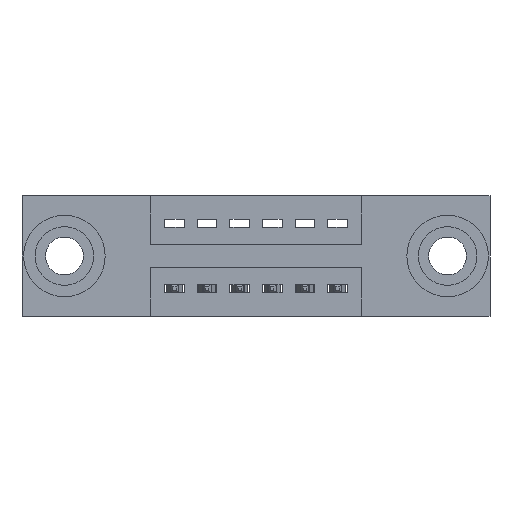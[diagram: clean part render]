
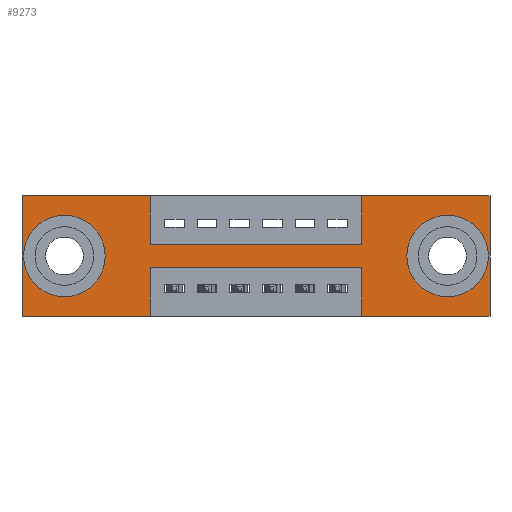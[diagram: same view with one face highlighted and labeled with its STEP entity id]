
A CAD part, front view. The second image highlights one B-rep face of the part: STEP entity #9273.
In plain terms, the highlighted planar face has unit normal (0, -1, 0).
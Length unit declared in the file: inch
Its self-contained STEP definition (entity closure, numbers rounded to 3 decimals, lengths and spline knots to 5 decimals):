
#13 = EDGE_CURVE ( 'NONE', #6455, #7511, #6539, .T. ) ;
#36 = ORIENTED_EDGE ( 'NONE', *, *, #2838, .F. ) ;
#334 = ORIENTED_EDGE ( 'NONE', *, *, #9604, .F. ) ;
#402 = DIRECTION ( 'NONE',  ( -1., 0., 0. ) ) ;
#462 = CARTESIAN_POINT ( 'NONE',  ( 0.3925, 0., -0.22 ) ) ;
#620 = EDGE_CURVE ( 'NONE', #8807, #6455, #6521, .T. ) ;
#662 = CIRCLE ( 'NONE', #8986, 0.078 ) ;
#701 = CARTESIAN_POINT ( 'NONE',  ( 1.435, 0., 0. ) ) ;
#770 = CIRCLE ( 'NONE', #5328, 0.078 ) ;
#779 = VERTEX_POINT ( 'NONE', #6749 ) ;
#894 = DIRECTION ( 'NONE',  ( 0., 1., 0. ) ) ;
#929 = VERTEX_POINT ( 'NONE', #1801 ) ;
#1000 = CARTESIAN_POINT ( 'NONE',  ( 0.3925, 0., -0.37 ) ) ;
#1002 = VECTOR ( 'NONE', #3045, 39.37008 ) ;
#1254 = DIRECTION ( 'NONE',  ( -1., 0., 0. ) ) ;
#1285 = CARTESIAN_POINT ( 'NONE',  ( 0.3925, 0., -0.22 ) ) ;
#1339 = LINE ( 'NONE', #2306, #7148 ) ;
#1533 = VECTOR ( 'NONE', #8848, 39.37008 ) ;
#1583 = CARTESIAN_POINT ( 'NONE',  ( 0.13, 0., -0.185 ) ) ;
#1602 = CARTESIAN_POINT ( 'NONE',  ( 0.3925, 0., 0. ) ) ;
#1707 = CIRCLE ( 'NONE', #4365, 0.078 ) ;
#1733 = ORIENTED_EDGE ( 'NONE', *, *, #6321, .F. ) ;
#1801 = CARTESIAN_POINT ( 'NONE',  ( 0.13, 0., -0.263 ) ) ;
#1841 = VECTOR ( 'NONE', #4592, 39.37008 ) ;
#2150 = DIRECTION ( 'NONE',  ( 0., 0., 1. ) ) ;
#2223 = DIRECTION ( 'NONE',  ( 1., 0., 0. ) ) ;
#2278 = EDGE_CURVE ( 'NONE', #3376, #7902, #6494, .T. ) ;
#2303 = ORIENTED_EDGE ( 'NONE', *, *, #620, .F. ) ;
#2306 = CARTESIAN_POINT ( 'NONE',  ( 0., 0., 0. ) ) ;
#2438 = CARTESIAN_POINT ( 'NONE',  ( 1.0425, 0., -0.37 ) ) ;
#2489 = DIRECTION ( 'NONE',  ( 0., -1., 0. ) ) ;
#2540 = CARTESIAN_POINT ( 'NONE',  ( 1.305, 0., -0.107 ) ) ;
#2641 = VERTEX_POINT ( 'NONE', #2540 ) ;
#2838 = EDGE_CURVE ( 'NONE', #8571, #8807, #6844, .T. ) ;
#3045 = DIRECTION ( 'NONE',  ( 0., 0., -1. ) ) ;
#3349 = VECTOR ( 'NONE', #6826, 39.37008 ) ;
#3357 = DIRECTION ( 'NONE',  ( 0., 0., 1. ) ) ;
#3368 = VECTOR ( 'NONE', #402, 39.37008 ) ;
#3376 = VERTEX_POINT ( 'NONE', #1000 ) ;
#3563 = VERTEX_POINT ( 'NONE', #9970 ) ;
#3621 = EDGE_CURVE ( 'NONE', #6509, #5295, #8711, .T. ) ;
#3659 = VERTEX_POINT ( 'NONE', #2438 ) ;
#3682 = VECTOR ( 'NONE', #1254, 39.37008 ) ;
#3724 = CARTESIAN_POINT ( 'NONE',  ( 0.3925, 0., -0.15 ) ) ;
#3818 = ORIENTED_EDGE ( 'NONE', *, *, #7520, .F. ) ;
#3982 = CARTESIAN_POINT ( 'NONE',  ( 0., 0., -0.37 ) ) ;
#4071 = VECTOR ( 'NONE', #9124, 39.37008 ) ;
#4095 = DIRECTION ( 'NONE',  ( 0., 1., 0. ) ) ;
#4107 = DIRECTION ( 'NONE',  ( 0., 0., -1. ) ) ;
#4365 = AXIS2_PLACEMENT_3D ( 'NONE', #7969, #4095, #3357 ) ;
#4385 = LINE ( 'NONE', #3724, #5956 ) ;
#4532 = CARTESIAN_POINT ( 'NONE',  ( 1.435, 0., 0. ) ) ;
#4582 = DIRECTION ( 'NONE',  ( 0., 0., 1. ) ) ;
#4592 = DIRECTION ( 'NONE',  ( 1., 0., 0. ) ) ;
#4821 = PLANE ( 'NONE',  #5993 ) ;
#4945 = CARTESIAN_POINT ( 'NONE',  ( 0.3925, 0., -0.15 ) ) ;
#5007 = LINE ( 'NONE', #6432, #7918 ) ;
#5079 = LINE ( 'NONE', #6135, #7621 ) ;
#5278 = CARTESIAN_POINT ( 'NONE',  ( 0.3925, 0., 0. ) ) ;
#5281 = CARTESIAN_POINT ( 'NONE',  ( 1.0425, 0., -0.15 ) ) ;
#5295 = VERTEX_POINT ( 'NONE', #4945 ) ;
#5328 = AXIS2_PLACEMENT_3D ( 'NONE', #8374, #9921, #7552 ) ;
#5540 = AXIS2_PLACEMENT_3D ( 'NONE', #1583, #7005, #4582 ) ;
#5598 = DIRECTION ( 'NONE',  ( 0., 0., -1. ) ) ;
#5635 = CARTESIAN_POINT ( 'NONE',  ( 1.435, 0., -0.37 ) ) ;
#5852 = VERTEX_POINT ( 'NONE', #9153 ) ;
#5908 = LINE ( 'NONE', #462, #1533 ) ;
#5956 = VECTOR ( 'NONE', #2223, 39.37008 ) ;
#5993 = AXIS2_PLACEMENT_3D ( 'NONE', #3982, #2489, #5598 ) ;
#6012 = CARTESIAN_POINT ( 'NONE',  ( 0., 0., 0. ) ) ;
#6135 = CARTESIAN_POINT ( 'NONE',  ( 1.0425, 0., -0.37 ) ) ;
#6182 = ORIENTED_EDGE ( 'NONE', *, *, #9548, .F. ) ;
#6236 = CARTESIAN_POINT ( 'NONE',  ( 1.305, 0., -0.185 ) ) ;
#6321 = EDGE_CURVE ( 'NONE', #7511, #3659, #9897, .T. ) ;
#6374 = EDGE_CURVE ( 'NONE', #5295, #8571, #4385, .T. ) ;
#6392 = EDGE_CURVE ( 'NONE', #2641, #3563, #770, .T. ) ;
#6403 = CARTESIAN_POINT ( 'NONE',  ( 1.0425, 0., 0. ) ) ;
#6421 = CIRCLE ( 'NONE', #5540, 0.078 ) ;
#6432 = CARTESIAN_POINT ( 'NONE',  ( 0.3925, 0., -0.37 ) ) ;
#6455 = VERTEX_POINT ( 'NONE', #4532 ) ;
#6494 = LINE ( 'NONE', #7434, #3368 ) ;
#6509 = VERTEX_POINT ( 'NONE', #1602 ) ;
#6521 = LINE ( 'NONE', #8203, #6895 ) ;
#6528 = EDGE_CURVE ( 'NONE', #3563, #2641, #662, .T. ) ;
#6539 = LINE ( 'NONE', #701, #1002 ) ;
#6556 = EDGE_LOOP ( 'NONE', ( #3818, #6182, #334, #1733, #8429, #2303, #36, #8124, #10021, #8700, #9625, #8661 ) ) ;
#6749 = CARTESIAN_POINT ( 'NONE',  ( 1.0425, 0., -0.22 ) ) ;
#6758 = FACE_BOUND ( 'NONE', #9317, .T. ) ;
#6826 = DIRECTION ( 'NONE',  ( 0., 0., -1. ) ) ;
#6844 = LINE ( 'NONE', #9515, #4071 ) ;
#6895 = VECTOR ( 'NONE', #7303, 39.37008 ) ;
#7005 = DIRECTION ( 'NONE',  ( 0., 1., 0. ) ) ;
#7148 = VECTOR ( 'NONE', #9240, 39.37008 ) ;
#7189 = ORIENTED_EDGE ( 'NONE', *, *, #7844, .T. ) ;
#7243 = EDGE_CURVE ( 'NONE', #8866, #6509, #7813, .T. ) ;
#7303 = DIRECTION ( 'NONE',  ( 1., 0., 0. ) ) ;
#7380 = FACE_OUTER_BOUND ( 'NONE', #6556, .T. ) ;
#7434 = CARTESIAN_POINT ( 'NONE',  ( 0., 0., -0.37 ) ) ;
#7511 = VERTEX_POINT ( 'NONE', #5635 ) ;
#7520 = EDGE_CURVE ( 'NONE', #7986, #3376, #5007, .T. ) ;
#7552 = DIRECTION ( 'NONE',  ( 0., 0., -1. ) ) ;
#7621 = VECTOR ( 'NONE', #2150, 39.37008 ) ;
#7813 = LINE ( 'NONE', #6012, #1841 ) ;
#7844 = EDGE_CURVE ( 'NONE', #5852, #929, #6421, .T. ) ;
#7860 = DIRECTION ( 'NONE',  ( 0., 0., -1. ) ) ;
#7902 = VERTEX_POINT ( 'NONE', #7907 ) ;
#7907 = CARTESIAN_POINT ( 'NONE',  ( 0., 0., -0.37 ) ) ;
#7908 = EDGE_CURVE ( 'NONE', #929, #5852, #1707, .T. ) ;
#7918 = VECTOR ( 'NONE', #4107, 39.37008 ) ;
#7969 = CARTESIAN_POINT ( 'NONE',  ( 0.13, 0., -0.185 ) ) ;
#7986 = VERTEX_POINT ( 'NONE', #1285 ) ;
#8124 = ORIENTED_EDGE ( 'NONE', *, *, #6374, .F. ) ;
#8161 = ORIENTED_EDGE ( 'NONE', *, *, #6528, .T. ) ;
#8203 = CARTESIAN_POINT ( 'NONE',  ( 0., 0., 0. ) ) ;
#8232 = CARTESIAN_POINT ( 'NONE',  ( 0., 0., 0. ) ) ;
#8370 = FACE_BOUND ( 'NONE', #9298, .T. ) ;
#8374 = CARTESIAN_POINT ( 'NONE',  ( 1.305, 0., -0.185 ) ) ;
#8429 = ORIENTED_EDGE ( 'NONE', *, *, #13, .F. ) ;
#8498 = EDGE_CURVE ( 'NONE', #7902, #8866, #1339, .T. ) ;
#8559 = ORIENTED_EDGE ( 'NONE', *, *, #7908, .T. ) ;
#8571 = VERTEX_POINT ( 'NONE', #5281 ) ;
#8661 = ORIENTED_EDGE ( 'NONE', *, *, #2278, .F. ) ;
#8700 = ORIENTED_EDGE ( 'NONE', *, *, #7243, .F. ) ;
#8711 = LINE ( 'NONE', #5278, #3349 ) ;
#8807 = VERTEX_POINT ( 'NONE', #6403 ) ;
#8848 = DIRECTION ( 'NONE',  ( -1., 0., 0. ) ) ;
#8866 = VERTEX_POINT ( 'NONE', #8232 ) ;
#8986 = AXIS2_PLACEMENT_3D ( 'NONE', #6236, #894, #7860 ) ;
#9124 = DIRECTION ( 'NONE',  ( 0., 0., 1. ) ) ;
#9153 = CARTESIAN_POINT ( 'NONE',  ( 0.13, 0., -0.107 ) ) ;
#9240 = DIRECTION ( 'NONE',  ( 0., 0., 1. ) ) ;
#9273 = ADVANCED_FACE ( 'NONE', ( #6758, #8370, #7380 ), #4821, .T. ) ;
#9298 = EDGE_LOOP ( 'NONE', ( #7189, #8559 ) ) ;
#9317 = EDGE_LOOP ( 'NONE', ( #9382, #8161 ) ) ;
#9382 = ORIENTED_EDGE ( 'NONE', *, *, #6392, .T. ) ;
#9515 = CARTESIAN_POINT ( 'NONE',  ( 1.0425, 0., 0. ) ) ;
#9548 = EDGE_CURVE ( 'NONE', #779, #7986, #5908, .T. ) ;
#9604 = EDGE_CURVE ( 'NONE', #3659, #779, #5079, .T. ) ;
#9625 = ORIENTED_EDGE ( 'NONE', *, *, #8498, .F. ) ;
#9768 = CARTESIAN_POINT ( 'NONE',  ( 0., 0., -0.37 ) ) ;
#9897 = LINE ( 'NONE', #9768, #3682 ) ;
#9921 = DIRECTION ( 'NONE',  ( 0., 1., 0. ) ) ;
#9970 = CARTESIAN_POINT ( 'NONE',  ( 1.305, 0., -0.263 ) ) ;
#10021 = ORIENTED_EDGE ( 'NONE', *, *, #3621, .F. ) ;
